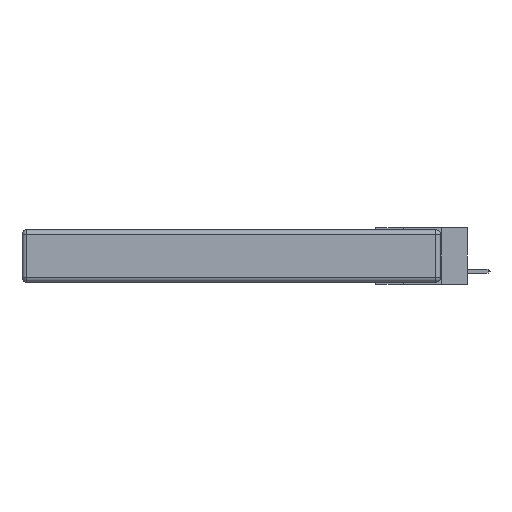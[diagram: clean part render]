
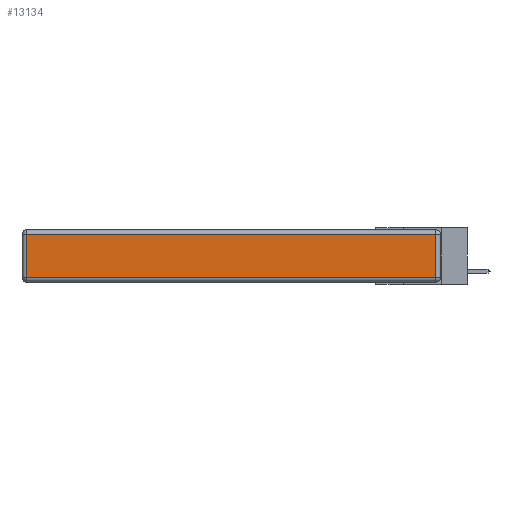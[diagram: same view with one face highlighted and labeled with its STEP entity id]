
A CAD part, left-side view. The second image highlights one B-rep face of the part: STEP entity #13134.
In plain terms, the highlighted planar face has unit normal (-1, 0, 0).
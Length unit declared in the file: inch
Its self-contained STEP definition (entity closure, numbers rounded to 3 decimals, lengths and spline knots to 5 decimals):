
#659 = ORIENTED_EDGE ( 'NONE', *, *, #9342, .T. ) ;
#694 = VECTOR ( 'NONE', #4403, 39.37008 ) ;
#1717 = DIRECTION ( 'NONE',  ( 0., 0., -1. ) ) ;
#2072 = CARTESIAN_POINT ( 'NONE',  ( 0., 0., -0.343 ) ) ;
#2136 = PLANE ( 'NONE',  #10851 ) ;
#2833 = CARTESIAN_POINT ( 'NONE',  ( 0., 2.72, -0.343 ) ) ;
#3032 = LINE ( 'NONE', #8545, #7978 ) ;
#3116 = ORIENTED_EDGE ( 'NONE', *, *, #6905, .T. ) ;
#3216 = EDGE_CURVE ( 'NONE', #9688, #9016, #5494, .T. ) ;
#3511 = VERTEX_POINT ( 'NONE', #13272 ) ;
#3532 = DIRECTION ( 'NONE',  ( -1., 0., 0. ) ) ;
#4403 = DIRECTION ( 'NONE',  ( 0., -1., 0. ) ) ;
#4701 = DIRECTION ( 'NONE',  ( 0., 0., 1. ) ) ;
#4827 = CARTESIAN_POINT ( 'NONE',  ( 0., 2.72, -0.03 ) ) ;
#5220 = LINE ( 'NONE', #2833, #13672 ) ;
#5494 = LINE ( 'NONE', #12243, #10997 ) ;
#6137 = DIRECTION ( 'NONE',  ( 0., 0., 1. ) ) ;
#6905 = EDGE_CURVE ( 'NONE', #10290, #3511, #7439, .T. ) ;
#7155 = DIRECTION ( 'NONE',  ( 0., 1., 0. ) ) ;
#7439 = LINE ( 'NONE', #10689, #694 ) ;
#7978 = VECTOR ( 'NONE', #6137, 39.37008 ) ;
#8545 = CARTESIAN_POINT ( 'NONE',  ( 0., 0.03, -0.343 ) ) ;
#8703 = CARTESIAN_POINT ( 'NONE',  ( 0., 2.72, -0.313 ) ) ;
#9016 = VERTEX_POINT ( 'NONE', #4827 ) ;
#9256 = FACE_OUTER_BOUND ( 'NONE', #9604, .T. ) ;
#9342 = EDGE_CURVE ( 'NONE', #9016, #10290, #5220, .T. ) ;
#9429 = CARTESIAN_POINT ( 'NONE',  ( 0., 0.03, -0.03 ) ) ;
#9604 = EDGE_LOOP ( 'NONE', ( #3116, #12457, #13005, #659 ) ) ;
#9688 = VERTEX_POINT ( 'NONE', #9429 ) ;
#10161 = EDGE_CURVE ( 'NONE', #3511, #9688, #3032, .T. ) ;
#10290 = VERTEX_POINT ( 'NONE', #8703 ) ;
#10689 = CARTESIAN_POINT ( 'NONE',  ( 0., 0., -0.313 ) ) ;
#10851 = AXIS2_PLACEMENT_3D ( 'NONE', #2072, #3532, #4701 ) ;
#10997 = VECTOR ( 'NONE', #7155, 39.37008 ) ;
#12243 = CARTESIAN_POINT ( 'NONE',  ( 0., 2.75, -0.03 ) ) ;
#12457 = ORIENTED_EDGE ( 'NONE', *, *, #10161, .T. ) ;
#13005 = ORIENTED_EDGE ( 'NONE', *, *, #3216, .T. ) ;
#13134 = ADVANCED_FACE ( 'NONE', ( #9256 ), #2136, .T. ) ;
#13272 = CARTESIAN_POINT ( 'NONE',  ( 0., 0.03, -0.313 ) ) ;
#13672 = VECTOR ( 'NONE', #1717, 39.37008 ) ;
